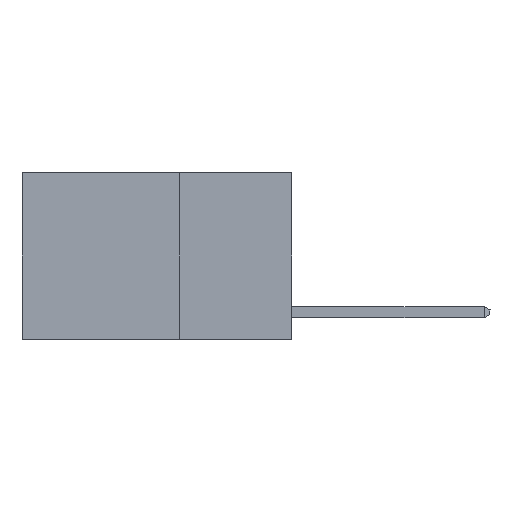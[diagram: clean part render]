
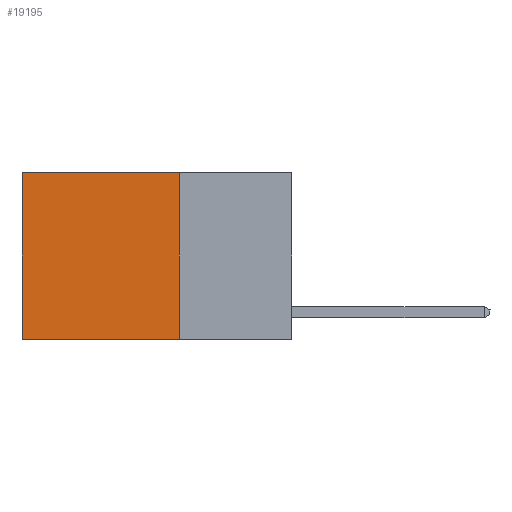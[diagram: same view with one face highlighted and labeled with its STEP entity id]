
A CAD part, left-side view. The second image highlights one B-rep face of the part: STEP entity #19195.
In plain terms, the highlighted planar face has unit normal (-1, 0, 0).
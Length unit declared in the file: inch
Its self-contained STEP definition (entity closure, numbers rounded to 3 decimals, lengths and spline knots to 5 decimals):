
#992 = ORIENTED_EDGE ( 'NONE', *, *, #23874, .T. ) ;
#1487 = LINE ( 'NONE', #3756, #12588 ) ;
#2690 = EDGE_CURVE ( 'NONE', #17466, #22825, #15557, .T. ) ;
#3756 = CARTESIAN_POINT ( 'NONE',  ( 0.2625, 0.6, 0. ) ) ;
#4995 = ORIENTED_EDGE ( 'NONE', *, *, #19186, .T. ) ;
#5820 = CARTESIAN_POINT ( 'NONE',  ( 0.2625, 0.25, -0.37 ) ) ;
#5908 = VERTEX_POINT ( 'NONE', #10217 ) ;
#7453 = CARTESIAN_POINT ( 'NONE',  ( 0.2625, 0.25, 0. ) ) ;
#9084 = CARTESIAN_POINT ( 'NONE',  ( 0.2625, 0.25, -0.37 ) ) ;
#9222 = DIRECTION ( 'NONE',  ( 0., 0., -1. ) ) ;
#10217 = CARTESIAN_POINT ( 'NONE',  ( 0.2625, 0.25, 0. ) ) ;
#10433 = CARTESIAN_POINT ( 'NONE',  ( 0.2625, 0.25, 0. ) ) ;
#11309 = VECTOR ( 'NONE', #22790, 39.37008 ) ;
#12588 = VECTOR ( 'NONE', #16946, 39.37008 ) ;
#14854 = DIRECTION ( 'NONE',  ( 0., 0., -1. ) ) ;
#15008 = CARTESIAN_POINT ( 'NONE',  ( 0.2625, 0.6, 0. ) ) ;
#15557 = LINE ( 'NONE', #5820, #20021 ) ;
#16946 = DIRECTION ( 'NONE',  ( 0., 0., -1. ) ) ;
#17466 = VERTEX_POINT ( 'NONE', #9084 ) ;
#17950 = VERTEX_POINT ( 'NONE', #15008 ) ;
#18411 = FACE_OUTER_BOUND ( 'NONE', #18699, .T. ) ;
#18699 = EDGE_LOOP ( 'NONE', ( #4995, #19910, #22087, #992 ) ) ;
#19186 = EDGE_CURVE ( 'NONE', #17950, #22825, #1487, .T. ) ;
#19195 = ADVANCED_FACE ( 'NONE', ( #18411 ), #23537, .F. ) ;
#19910 = ORIENTED_EDGE ( 'NONE', *, *, #2690, .F. ) ;
#20000 = AXIS2_PLACEMENT_3D ( 'NONE', #10433, #27910, #14854 ) ;
#20021 = VECTOR ( 'NONE', #21179, 39.37008 ) ;
#20162 = CARTESIAN_POINT ( 'NONE',  ( 0.2625, 0.25, 0. ) ) ;
#21179 = DIRECTION ( 'NONE',  ( 0., 1., 0. ) ) ;
#22087 = ORIENTED_EDGE ( 'NONE', *, *, #22601, .F. ) ;
#22257 = LINE ( 'NONE', #7453, #11309 ) ;
#22601 = EDGE_CURVE ( 'NONE', #5908, #17466, #25066, .T. ) ;
#22790 = DIRECTION ( 'NONE',  ( 0., 1., 0. ) ) ;
#22825 = VERTEX_POINT ( 'NONE', #25391 ) ;
#23537 = PLANE ( 'NONE',  #20000 ) ;
#23690 = VECTOR ( 'NONE', #9222, 39.37008 ) ;
#23874 = EDGE_CURVE ( 'NONE', #5908, #17950, #22257, .T. ) ;
#25066 = LINE ( 'NONE', #20162, #23690 ) ;
#25391 = CARTESIAN_POINT ( 'NONE',  ( 0.2625, 0.6, -0.37 ) ) ;
#27910 = DIRECTION ( 'NONE',  ( 1., 0., 0. ) ) ;
